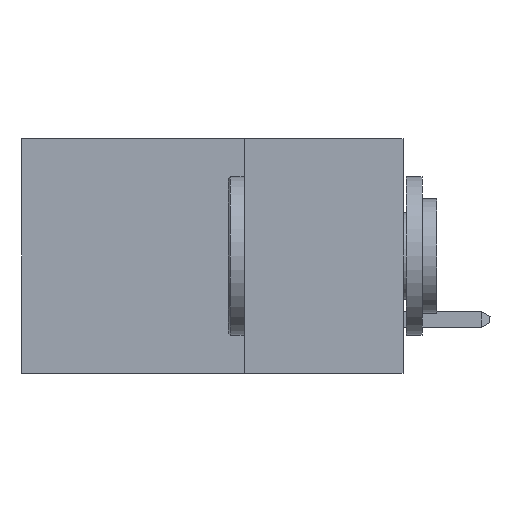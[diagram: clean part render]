
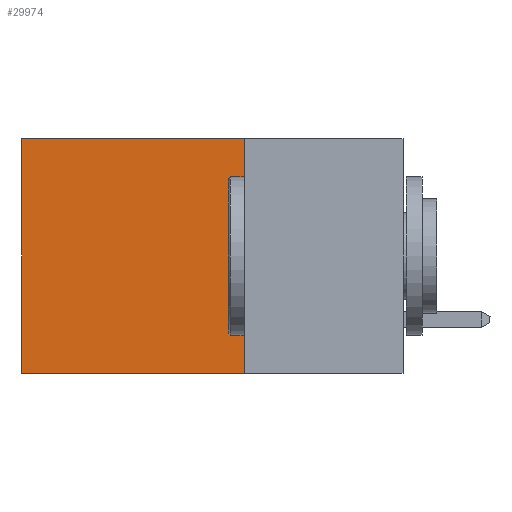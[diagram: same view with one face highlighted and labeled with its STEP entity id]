
A CAD part, left-side view. The second image highlights one B-rep face of the part: STEP entity #29974.
In plain terms, the highlighted planar face has unit normal (-1, 0, 0).
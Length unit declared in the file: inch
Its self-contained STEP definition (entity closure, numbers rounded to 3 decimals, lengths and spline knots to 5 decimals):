
#447 = CARTESIAN_POINT ( 'NONE',  ( 0.2875, 0.25, -0.37 ) ) ;
#1253 = DIRECTION ( 'NONE',  ( 0., 0., -1. ) ) ;
#1417 = ORIENTED_EDGE ( 'NONE', *, *, #17728, .T. ) ;
#1577 = LINE ( 'NONE', #5444, #17132 ) ;
#1662 = CARTESIAN_POINT ( 'NONE',  ( 0.2875, 0.6, 0. ) ) ;
#3000 = ORIENTED_EDGE ( 'NONE', *, *, #18114, .F. ) ;
#3960 = VECTOR ( 'NONE', #17545, 39.37008 ) ;
#5444 = CARTESIAN_POINT ( 'NONE',  ( 0.2875, 0.25, 0. ) ) ;
#6042 = VECTOR ( 'NONE', #13948, 39.37008 ) ;
#6543 = PLANE ( 'NONE',  #22325 ) ;
#6805 = ORIENTED_EDGE ( 'NONE', *, *, #31674, .F. ) ;
#9048 = VERTEX_POINT ( 'NONE', #22567 ) ;
#9159 = DIRECTION ( 'NONE',  ( 0., 0., -1. ) ) ;
#11038 = VECTOR ( 'NONE', #30108, 39.37008 ) ;
#13393 = LINE ( 'NONE', #447, #11038 ) ;
#13948 = DIRECTION ( 'NONE',  ( 0., 0., -1. ) ) ;
#14408 = EDGE_CURVE ( 'NONE', #14842, #27075, #15011, .T. ) ;
#14842 = VERTEX_POINT ( 'NONE', #1662 ) ;
#15011 = LINE ( 'NONE', #24218, #6042 ) ;
#15972 = DIRECTION ( 'NONE',  ( 1., 0., 0. ) ) ;
#17132 = VECTOR ( 'NONE', #1253, 39.37008 ) ;
#17545 = DIRECTION ( 'NONE',  ( 0., 1., 0. ) ) ;
#17728 = EDGE_CURVE ( 'NONE', #28016, #14842, #19904, .T. ) ;
#18114 = EDGE_CURVE ( 'NONE', #28016, #9048, #1577, .T. ) ;
#19721 = CARTESIAN_POINT ( 'NONE',  ( 0.2875, 0.6, -0.37 ) ) ;
#19904 = LINE ( 'NONE', #20144, #3960 ) ;
#20144 = CARTESIAN_POINT ( 'NONE',  ( 0.2875, 0.25, 0. ) ) ;
#20692 = CARTESIAN_POINT ( 'NONE',  ( 0.2875, 0.25, 0. ) ) ;
#22325 = AXIS2_PLACEMENT_3D ( 'NONE', #30888, #15972, #9159 ) ;
#22567 = CARTESIAN_POINT ( 'NONE',  ( 0.2875, 0.25, -0.37 ) ) ;
#24007 = FACE_OUTER_BOUND ( 'NONE', #28691, .T. ) ;
#24218 = CARTESIAN_POINT ( 'NONE',  ( 0.2875, 0.6, 0. ) ) ;
#27075 = VERTEX_POINT ( 'NONE', #19721 ) ;
#27653 = ORIENTED_EDGE ( 'NONE', *, *, #14408, .T. ) ;
#28016 = VERTEX_POINT ( 'NONE', #20692 ) ;
#28691 = EDGE_LOOP ( 'NONE', ( #27653, #6805, #3000, #1417 ) ) ;
#29974 = ADVANCED_FACE ( 'NONE', ( #24007 ), #6543, .F. ) ;
#30108 = DIRECTION ( 'NONE',  ( 0., 1., 0. ) ) ;
#30888 = CARTESIAN_POINT ( 'NONE',  ( 0.2875, 0.25, 0. ) ) ;
#31674 = EDGE_CURVE ( 'NONE', #9048, #27075, #13393, .T. ) ;
